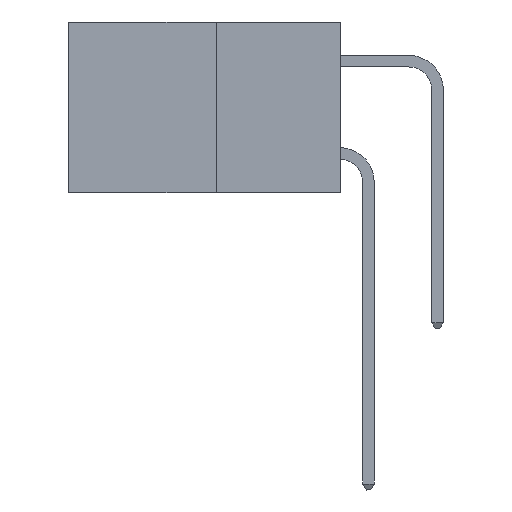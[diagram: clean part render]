
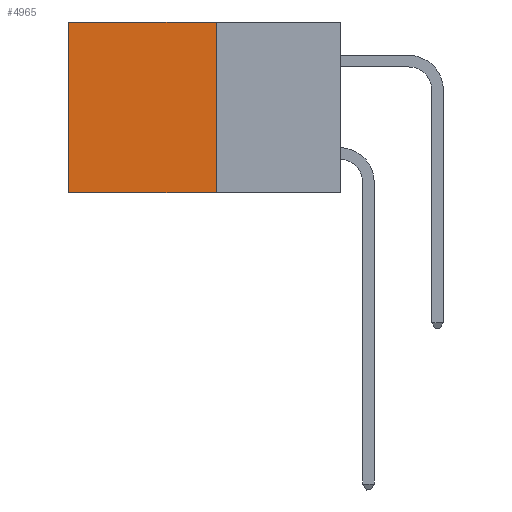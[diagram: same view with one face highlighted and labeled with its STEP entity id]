
A CAD part, left-side view. The second image highlights one B-rep face of the part: STEP entity #4965.
In plain terms, the highlighted planar face has unit normal (-1, 0, 0).
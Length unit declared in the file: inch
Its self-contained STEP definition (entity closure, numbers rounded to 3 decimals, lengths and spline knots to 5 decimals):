
#1109 = LINE ( 'NONE', #16543, #24039 ) ;
#1584 = EDGE_CURVE ( 'NONE', #24782, #13550, #1109, .T. ) ;
#1715 = CARTESIAN_POINT ( 'NONE',  ( 0.277, 0.27, -0.37 ) ) ;
#1756 = VECTOR ( 'NONE', #4430, 39.37008 ) ;
#2341 = ORIENTED_EDGE ( 'NONE', *, *, #1584, .T. ) ;
#2447 = EDGE_CURVE ( 'NONE', #25780, #26394, #24697, .T. ) ;
#2671 = VECTOR ( 'NONE', #6103, 39.37008 ) ;
#4430 = DIRECTION ( 'NONE',  ( 0., 0., -1. ) ) ;
#4474 = DIRECTION ( 'NONE',  ( 0., 1., 0. ) ) ;
#4965 = ADVANCED_FACE ( 'NONE', ( #27782 ), #21808, .F. ) ;
#6103 = DIRECTION ( 'NONE',  ( 0., 1., 0. ) ) ;
#6167 = CARTESIAN_POINT ( 'NONE',  ( 0.277, 0.27, 0. ) ) ;
#7711 = EDGE_CURVE ( 'NONE', #25780, #24782, #20375, .T. ) ;
#7960 = LINE ( 'NONE', #19939, #20402 ) ;
#11345 = CARTESIAN_POINT ( 'NONE',  ( 0.277, 0.59, -0.37 ) ) ;
#12058 = EDGE_CURVE ( 'NONE', #26394, #13550, #7960, .T. ) ;
#13550 = VERTEX_POINT ( 'NONE', #11345 ) ;
#15673 = ORIENTED_EDGE ( 'NONE', *, *, #7711, .T. ) ;
#16468 = ORIENTED_EDGE ( 'NONE', *, *, #12058, .F. ) ;
#16543 = CARTESIAN_POINT ( 'NONE',  ( 0.277, 0.59, -0.37 ) ) ;
#16919 = ORIENTED_EDGE ( 'NONE', *, *, #2447, .F. ) ;
#17756 = AXIS2_PLACEMENT_3D ( 'NONE', #21996, #21770, #21697 ) ;
#18660 = DIRECTION ( 'NONE',  ( 0., 0., -1. ) ) ;
#19939 = CARTESIAN_POINT ( 'NONE',  ( 0.277, 0.27, -0.37 ) ) ;
#20375 = LINE ( 'NONE', #6167, #2671 ) ;
#20402 = VECTOR ( 'NONE', #4474, 39.37008 ) ;
#21697 = DIRECTION ( 'NONE',  ( 0., 0., -1. ) ) ;
#21770 = DIRECTION ( 'NONE',  ( 1., 0., 0. ) ) ;
#21808 = PLANE ( 'NONE',  #17756 ) ;
#21831 = CARTESIAN_POINT ( 'NONE',  ( 0.277, 0.27, -0.37 ) ) ;
#21996 = CARTESIAN_POINT ( 'NONE',  ( 0.277, 0.27, -0.37 ) ) ;
#24039 = VECTOR ( 'NONE', #18660, 39.37008 ) ;
#24365 = CARTESIAN_POINT ( 'NONE',  ( 0.277, 0.27, 0. ) ) ;
#24697 = LINE ( 'NONE', #21831, #1756 ) ;
#24782 = VERTEX_POINT ( 'NONE', #25579 ) ;
#25579 = CARTESIAN_POINT ( 'NONE',  ( 0.277, 0.59, 0. ) ) ;
#25780 = VERTEX_POINT ( 'NONE', #24365 ) ;
#26394 = VERTEX_POINT ( 'NONE', #1715 ) ;
#27782 = FACE_OUTER_BOUND ( 'NONE', #27783, .T. ) ;
#27783 = EDGE_LOOP ( 'NONE', ( #2341, #16468, #16919, #15673 ) ) ;
